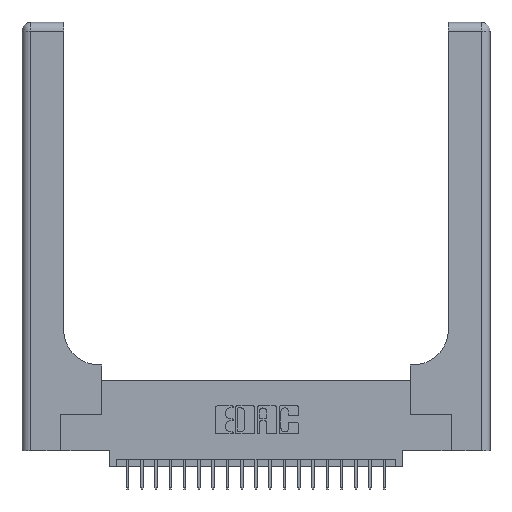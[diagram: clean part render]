
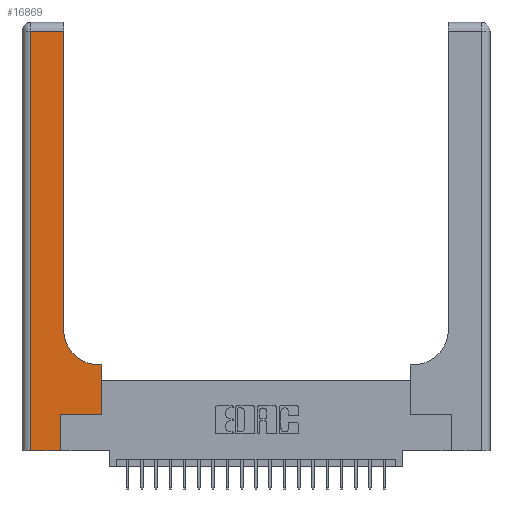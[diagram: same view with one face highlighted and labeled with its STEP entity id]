
A CAD part, top view. The second image highlights one B-rep face of the part: STEP entity #16869.
In plain terms, the highlighted planar face has unit normal (0, 0, 1).
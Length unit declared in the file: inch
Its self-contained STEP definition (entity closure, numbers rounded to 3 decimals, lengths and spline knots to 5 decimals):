
#520 = CARTESIAN_POINT ( 'NONE',  ( 0.2915, 0.85, 0.37 ) ) ;
#855 = DIRECTION ( 'NONE',  ( -1., 0., 0. ) ) ;
#1073 = LINE ( 'NONE', #10271, #14916 ) ;
#1149 = DIRECTION ( 'NONE',  ( 0., 0., -1. ) ) ;
#1348 = AXIS2_PLACEMENT_3D ( 'NONE', #2807, #1149, #855 ) ;
#1441 = AXIS2_PLACEMENT_3D ( 'NONE', #15735, #1446, #3180 ) ;
#1446 = DIRECTION ( 'NONE',  ( 0., 0., -1. ) ) ;
#2020 = EDGE_LOOP ( 'NONE', ( #20574, #14707, #13602, #11465, #2236, #8407, #8381, #10918, #21141 ) ) ;
#2186 = EDGE_CURVE ( 'NONE', #16546, #15195, #21837, .T. ) ;
#2236 = ORIENTED_EDGE ( 'NONE', *, *, #7870, .T. ) ;
#2654 = PLANE ( 'NONE',  #1348 ) ;
#2807 = CARTESIAN_POINT ( 'NONE',  ( 0., 3., 0.37 ) ) ;
#3180 = DIRECTION ( 'NONE',  ( 1., 0., 0. ) ) ;
#3307 = CARTESIAN_POINT ( 'NONE',  ( 0.269, 0.25, 0.37 ) ) ;
#3317 = VERTEX_POINT ( 'NONE', #7927 ) ;
#3653 = VECTOR ( 'NONE', #22071, 39.37008 ) ;
#3658 = VERTEX_POINT ( 'NONE', #21982 ) ;
#4695 = VERTEX_POINT ( 'NONE', #3307 ) ;
#5029 = EDGE_CURVE ( 'NONE', #4695, #18993, #9905, .T. ) ;
#5960 = VECTOR ( 'NONE', #11578, 39.37008 ) ;
#6103 = VECTOR ( 'NONE', #9295, 39.37008 ) ;
#6572 = EDGE_CURVE ( 'NONE', #3658, #3317, #10385, .T. ) ;
#6754 = EDGE_CURVE ( 'NONE', #16799, #11820, #1073, .T. ) ;
#7154 = CARTESIAN_POINT ( 'NONE',  ( 0.5585, 0.6, 0.37 ) ) ;
#7335 = DIRECTION ( 'NONE',  ( 0., 1., 0. ) ) ;
#7557 = CARTESIAN_POINT ( 'NONE',  ( 0.269, 0., 0.37 ) ) ;
#7870 = EDGE_CURVE ( 'NONE', #3317, #4695, #17663, .T. ) ;
#7927 = CARTESIAN_POINT ( 'NONE',  ( 0.269, 0., 0.37 ) ) ;
#8304 = CARTESIAN_POINT ( 'NONE',  ( 0.06, 3., 0.37 ) ) ;
#8381 = ORIENTED_EDGE ( 'NONE', *, *, #12924, .T. ) ;
#8394 = LINE ( 'NONE', #16548, #11775 ) ;
#8407 = ORIENTED_EDGE ( 'NONE', *, *, #5029, .T. ) ;
#9295 = DIRECTION ( 'NONE',  ( 0., 1., 0. ) ) ;
#9513 = CARTESIAN_POINT ( 'NONE',  ( 0.06, 2.94, 0.37 ) ) ;
#9755 = CARTESIAN_POINT ( 'NONE',  ( 0.269, 0.25, 0.37 ) ) ;
#9905 = LINE ( 'NONE', #9755, #5960 ) ;
#9962 = CARTESIAN_POINT ( 'NONE',  ( 0., 0., 0.37 ) ) ;
#10271 = CARTESIAN_POINT ( 'NONE',  ( 0., 2.94, 0.37 ) ) ;
#10356 = LINE ( 'NONE', #16556, #13454 ) ;
#10385 = LINE ( 'NONE', #9962, #11816 ) ;
#10846 = EDGE_CURVE ( 'NONE', #11820, #3658, #16371, .T. ) ;
#10918 = ORIENTED_EDGE ( 'NONE', *, *, #11319, .T. ) ;
#11319 = EDGE_CURVE ( 'NONE', #17296, #16546, #14089, .T. ) ;
#11465 = ORIENTED_EDGE ( 'NONE', *, *, #6572, .T. ) ;
#11578 = DIRECTION ( 'NONE',  ( 1., 0., 0. ) ) ;
#11775 = VECTOR ( 'NONE', #7335, 39.37008 ) ;
#11811 = CARTESIAN_POINT ( 'NONE',  ( 0.5585, 0.25, 0.37 ) ) ;
#11816 = VECTOR ( 'NONE', #20461, 39.37008 ) ;
#11820 = VERTEX_POINT ( 'NONE', #9513 ) ;
#12436 = VECTOR ( 'NONE', #19163, 39.37008 ) ;
#12924 = EDGE_CURVE ( 'NONE', #18993, #17296, #10356, .T. ) ;
#13090 = FACE_OUTER_BOUND ( 'NONE', #2020, .T. ) ;
#13454 = VECTOR ( 'NONE', #18366, 39.37008 ) ;
#13577 = DIRECTION ( 'NONE',  ( -1., 0., 0. ) ) ;
#13602 = ORIENTED_EDGE ( 'NONE', *, *, #10846, .T. ) ;
#14089 = LINE ( 'NONE', #20340, #3653 ) ;
#14707 = ORIENTED_EDGE ( 'NONE', *, *, #6754, .T. ) ;
#14916 = VECTOR ( 'NONE', #13577, 39.37008 ) ;
#15195 = VERTEX_POINT ( 'NONE', #520 ) ;
#15735 = CARTESIAN_POINT ( 'NONE',  ( 0.5415, 0.85, 0.37 ) ) ;
#16371 = LINE ( 'NONE', #8304, #12436 ) ;
#16546 = VERTEX_POINT ( 'NONE', #17895 ) ;
#16548 = CARTESIAN_POINT ( 'NONE',  ( 0.2915, 3., 0.37 ) ) ;
#16556 = CARTESIAN_POINT ( 'NONE',  ( 0.5585, 0.25, 0.37 ) ) ;
#16799 = VERTEX_POINT ( 'NONE', #18528 ) ;
#16869 = ADVANCED_FACE ( 'NONE', ( #13090 ), #2654, .F. ) ;
#17296 = VERTEX_POINT ( 'NONE', #7154 ) ;
#17663 = LINE ( 'NONE', #7557, #6103 ) ;
#17895 = CARTESIAN_POINT ( 'NONE',  ( 0.5415, 0.6, 0.37 ) ) ;
#18366 = DIRECTION ( 'NONE',  ( 0., 1., 0. ) ) ;
#18528 = CARTESIAN_POINT ( 'NONE',  ( 0.2915, 2.94, 0.37 ) ) ;
#18993 = VERTEX_POINT ( 'NONE', #11811 ) ;
#19163 = DIRECTION ( 'NONE',  ( 0., -1., 0. ) ) ;
#20340 = CARTESIAN_POINT ( 'NONE',  ( 0.2915, 0.6, 0.37 ) ) ;
#20461 = DIRECTION ( 'NONE',  ( 1., 0., 0. ) ) ;
#20574 = ORIENTED_EDGE ( 'NONE', *, *, #21596, .T. ) ;
#21141 = ORIENTED_EDGE ( 'NONE', *, *, #2186, .T. ) ;
#21596 = EDGE_CURVE ( 'NONE', #15195, #16799, #8394, .T. ) ;
#21837 = CIRCLE ( 'NONE', #1441, 0.25 ) ;
#21982 = CARTESIAN_POINT ( 'NONE',  ( 0.06, 0., 0.37 ) ) ;
#22071 = DIRECTION ( 'NONE',  ( -1., 0., 0. ) ) ;
